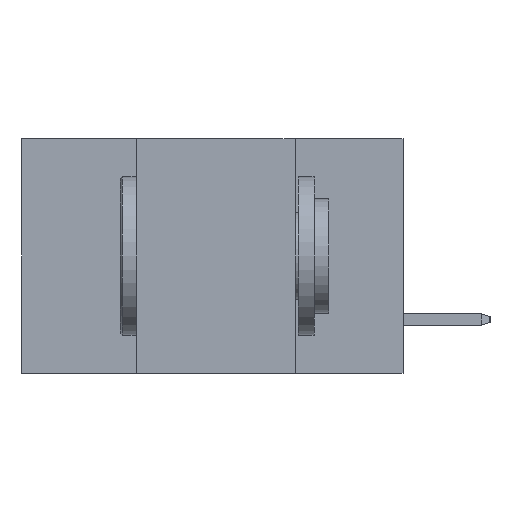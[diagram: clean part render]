
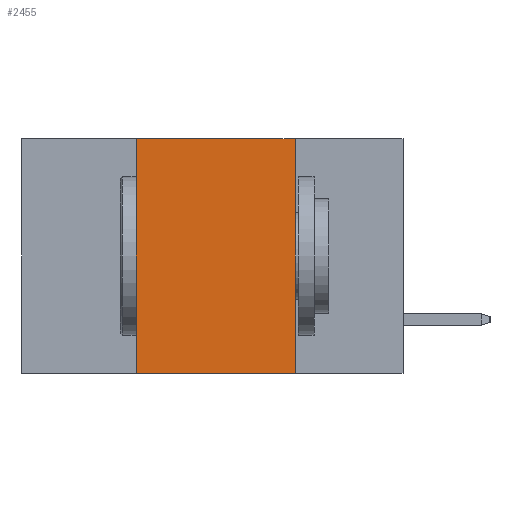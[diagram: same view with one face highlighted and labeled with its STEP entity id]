
A CAD part, left-side view. The second image highlights one B-rep face of the part: STEP entity #2455.
In plain terms, the highlighted planar face has unit normal (-1, 0, 0).
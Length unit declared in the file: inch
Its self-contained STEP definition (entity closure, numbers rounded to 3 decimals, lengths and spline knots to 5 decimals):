
#19 = CARTESIAN_POINT ( 'NONE',  ( 0., 0.17, 0. ) ) ;
#1741 = EDGE_LOOP ( 'NONE', ( #11647, #4863, #15510, #19987 ) ) ;
#2103 = DIRECTION ( 'NONE',  ( 0., 0., -1. ) ) ;
#2455 = ADVANCED_FACE ( 'NONE', ( #9604 ), #11937, .F. ) ;
#3082 = AXIS2_PLACEMENT_3D ( 'NONE', #13626, #17533, #15451 ) ;
#3468 = EDGE_CURVE ( 'NONE', #19062, #19773, #21603, .T. ) ;
#4459 = EDGE_CURVE ( 'NONE', #20194, #19773, #22685, .T. ) ;
#4863 = ORIENTED_EDGE ( 'NONE', *, *, #11799, .F. ) ;
#6312 = DIRECTION ( 'NONE',  ( 0., -1., 0. ) ) ;
#6495 = CARTESIAN_POINT ( 'NONE',  ( 0., 0.6, 0. ) ) ;
#9604 = FACE_OUTER_BOUND ( 'NONE', #1741, .T. ) ;
#10988 = CARTESIAN_POINT ( 'NONE',  ( 0., 0.42, -0.37 ) ) ;
#11647 = ORIENTED_EDGE ( 'NONE', *, *, #3468, .F. ) ;
#11799 = EDGE_CURVE ( 'NONE', #14339, #19062, #12957, .T. ) ;
#11937 = PLANE ( 'NONE',  #3082 ) ;
#12446 = DIRECTION ( 'NONE',  ( 0., -1., 0. ) ) ;
#12542 = EDGE_CURVE ( 'NONE', #20194, #14339, #20293, .T. ) ;
#12957 = LINE ( 'NONE', #6495, #13152 ) ;
#13152 = VECTOR ( 'NONE', #12446, 39.37008 ) ;
#13626 = CARTESIAN_POINT ( 'NONE',  ( 0., 0.6, 0. ) ) ;
#14339 = VERTEX_POINT ( 'NONE', #22621 ) ;
#15451 = DIRECTION ( 'NONE',  ( 0., 0., -1. ) ) ;
#15510 = ORIENTED_EDGE ( 'NONE', *, *, #12542, .F. ) ;
#16417 = CARTESIAN_POINT ( 'NONE',  ( 0., 0.6, -0.37 ) ) ;
#16933 = VECTOR ( 'NONE', #18208, 39.37008 ) ;
#17533 = DIRECTION ( 'NONE',  ( 1., 0., 0. ) ) ;
#18208 = DIRECTION ( 'NONE',  ( 0., 0., 1. ) ) ;
#19062 = VERTEX_POINT ( 'NONE', #19 ) ;
#19773 = VERTEX_POINT ( 'NONE', #20906 ) ;
#19987 = ORIENTED_EDGE ( 'NONE', *, *, #4459, .T. ) ;
#20194 = VERTEX_POINT ( 'NONE', #10988 ) ;
#20293 = LINE ( 'NONE', #24070, #16933 ) ;
#20906 = CARTESIAN_POINT ( 'NONE',  ( 0., 0.17, -0.37 ) ) ;
#21603 = LINE ( 'NONE', #23811, #23049 ) ;
#22621 = CARTESIAN_POINT ( 'NONE',  ( 0., 0.42, 0. ) ) ;
#22685 = LINE ( 'NONE', #16417, #24732 ) ;
#23049 = VECTOR ( 'NONE', #2103, 39.37008 ) ;
#23811 = CARTESIAN_POINT ( 'NONE',  ( 0., 0.17, 0. ) ) ;
#24070 = CARTESIAN_POINT ( 'NONE',  ( 0., 0.42, 0. ) ) ;
#24732 = VECTOR ( 'NONE', #6312, 39.37008 ) ;
